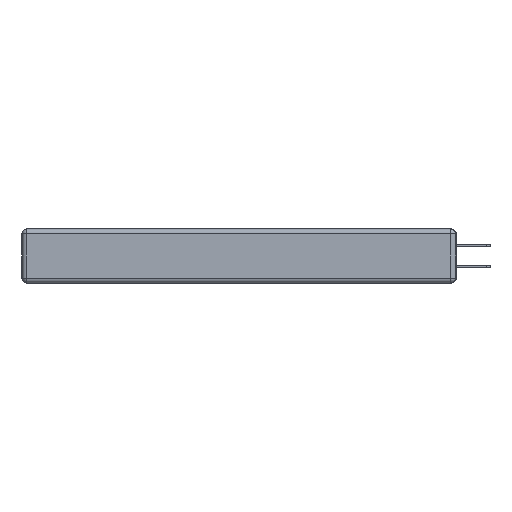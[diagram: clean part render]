
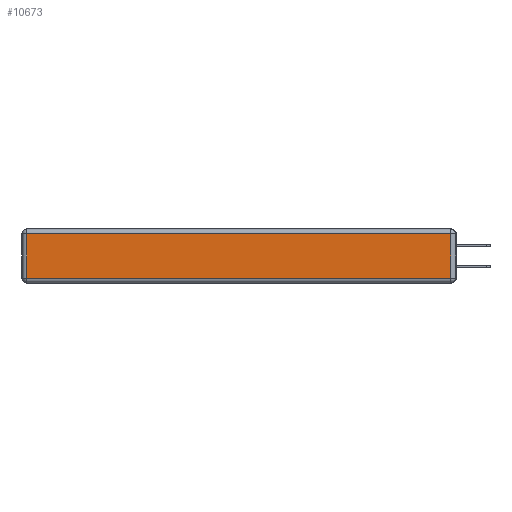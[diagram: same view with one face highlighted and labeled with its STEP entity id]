
A CAD part, left-side view. The second image highlights one B-rep face of the part: STEP entity #10673.
In plain terms, the highlighted planar face has unit normal (-1, 0, 0).
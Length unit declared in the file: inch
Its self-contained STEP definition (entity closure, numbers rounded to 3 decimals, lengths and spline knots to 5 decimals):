
#772 = LINE ( 'NONE', #11878, #6802 ) ;
#813 = ORIENTED_EDGE ( 'NONE', *, *, #7629, .T. ) ;
#1278 = VERTEX_POINT ( 'NONE', #12131 ) ;
#1734 = DIRECTION ( 'NONE',  ( 0., 0., -1. ) ) ;
#1786 = DIRECTION ( 'NONE',  ( -1., 0., 0. ) ) ;
#2102 = VERTEX_POINT ( 'NONE', #10955 ) ;
#2868 = CARTESIAN_POINT ( 'NONE',  ( 0., 0.03, -0.03 ) ) ;
#3761 = DIRECTION ( 'NONE',  ( 0., 0., 1. ) ) ;
#3831 = DIRECTION ( 'NONE',  ( 0., 0., 1. ) ) ;
#4450 = DIRECTION ( 'NONE',  ( 0., -1., 0. ) ) ;
#4536 = VERTEX_POINT ( 'NONE', #2868 ) ;
#4929 = ORIENTED_EDGE ( 'NONE', *, *, #8022, .T. ) ;
#6802 = VECTOR ( 'NONE', #1734, 39.37008 ) ;
#7629 = EDGE_CURVE ( 'NONE', #2102, #17999, #22817, .T. ) ;
#7928 = CARTESIAN_POINT ( 'NONE',  ( 0., 0.03, -0.313 ) ) ;
#8022 = EDGE_CURVE ( 'NONE', #4536, #1278, #10619, .T. ) ;
#8832 = CARTESIAN_POINT ( 'NONE',  ( 0., 0., -0.313 ) ) ;
#9324 = VECTOR ( 'NONE', #21289, 39.37008 ) ;
#10239 = EDGE_CURVE ( 'NONE', #17999, #4536, #17385, .T. ) ;
#10619 = LINE ( 'NONE', #21556, #9324 ) ;
#10673 = ADVANCED_FACE ( 'NONE', ( #21110 ), #12113, .T. ) ;
#10955 = CARTESIAN_POINT ( 'NONE',  ( 0., 2.72, -0.313 ) ) ;
#11878 = CARTESIAN_POINT ( 'NONE',  ( 0., 2.72, -0.343 ) ) ;
#12113 = PLANE ( 'NONE',  #19954 ) ;
#12131 = CARTESIAN_POINT ( 'NONE',  ( 0., 2.72, -0.03 ) ) ;
#12272 = EDGE_LOOP ( 'NONE', ( #813, #22041, #4929, #14078 ) ) ;
#14078 = ORIENTED_EDGE ( 'NONE', *, *, #14156, .T. ) ;
#14156 = EDGE_CURVE ( 'NONE', #1278, #2102, #772, .T. ) ;
#16778 = VECTOR ( 'NONE', #3761, 39.37008 ) ;
#17385 = LINE ( 'NONE', #21921, #16778 ) ;
#17485 = VECTOR ( 'NONE', #4450, 39.37008 ) ;
#17800 = CARTESIAN_POINT ( 'NONE',  ( 0., 0., -0.343 ) ) ;
#17999 = VERTEX_POINT ( 'NONE', #7928 ) ;
#19954 = AXIS2_PLACEMENT_3D ( 'NONE', #17800, #1786, #3831 ) ;
#21110 = FACE_OUTER_BOUND ( 'NONE', #12272, .T. ) ;
#21289 = DIRECTION ( 'NONE',  ( 0., 1., 0. ) ) ;
#21556 = CARTESIAN_POINT ( 'NONE',  ( 0., 2.75, -0.03 ) ) ;
#21921 = CARTESIAN_POINT ( 'NONE',  ( 0., 0.03, -0.343 ) ) ;
#22041 = ORIENTED_EDGE ( 'NONE', *, *, #10239, .T. ) ;
#22817 = LINE ( 'NONE', #8832, #17485 ) ;
